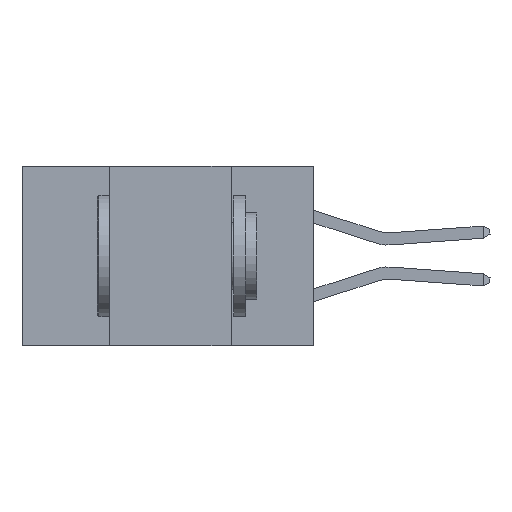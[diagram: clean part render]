
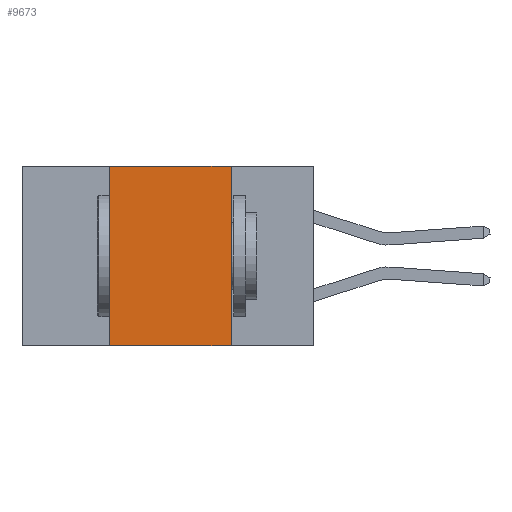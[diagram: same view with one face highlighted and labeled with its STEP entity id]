
A CAD part, left-side view. The second image highlights one B-rep face of the part: STEP entity #9673.
In plain terms, the highlighted planar face has unit normal (-1, 0, 0).
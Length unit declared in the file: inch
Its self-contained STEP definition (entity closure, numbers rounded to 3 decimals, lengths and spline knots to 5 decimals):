
#394 = VERTEX_POINT ( 'NONE', #27516 ) ;
#942 = ORIENTED_EDGE ( 'NONE', *, *, #21760, .F. ) ;
#1142 = DIRECTION ( 'NONE',  ( 1., 0., 0. ) ) ;
#1430 = DIRECTION ( 'NONE',  ( 0., 0., 1. ) ) ;
#1872 = ORIENTED_EDGE ( 'NONE', *, *, #23260, .F. ) ;
#2189 = DIRECTION ( 'NONE',  ( 0., -1., 0. ) ) ;
#4790 = LINE ( 'NONE', #5276, #15573 ) ;
#5215 = EDGE_CURVE ( 'NONE', #14139, #394, #22603, .T. ) ;
#5276 = CARTESIAN_POINT ( 'NONE',  ( 0., 0.6, 0. ) ) ;
#5800 = CARTESIAN_POINT ( 'NONE',  ( 0., 0.42, 0. ) ) ;
#5894 = LINE ( 'NONE', #25523, #15028 ) ;
#6830 = ORIENTED_EDGE ( 'NONE', *, *, #9731, .F. ) ;
#7863 = PLANE ( 'NONE',  #26238 ) ;
#9336 = VERTEX_POINT ( 'NONE', #13077 ) ;
#9538 = VERTEX_POINT ( 'NONE', #9573 ) ;
#9573 = CARTESIAN_POINT ( 'NONE',  ( 0., 0.42, 0. ) ) ;
#9673 = ADVANCED_FACE ( 'NONE', ( #17369 ), #7863, .F. ) ;
#9731 = EDGE_CURVE ( 'NONE', #14139, #9538, #24092, .T. ) ;
#11105 = VECTOR ( 'NONE', #2189, 39.37008 ) ;
#12783 = DIRECTION ( 'NONE',  ( 0., 0., -1. ) ) ;
#13077 = CARTESIAN_POINT ( 'NONE',  ( 0., 0.17, 0. ) ) ;
#14139 = VERTEX_POINT ( 'NONE', #23468 ) ;
#15028 = VECTOR ( 'NONE', #12783, 39.37008 ) ;
#15573 = VECTOR ( 'NONE', #17997, 39.37008 ) ;
#17369 = FACE_OUTER_BOUND ( 'NONE', #21183, .T. ) ;
#17784 = ORIENTED_EDGE ( 'NONE', *, *, #5215, .T. ) ;
#17997 = DIRECTION ( 'NONE',  ( 0., -1., 0. ) ) ;
#21183 = EDGE_LOOP ( 'NONE', ( #942, #1872, #6830, #17784 ) ) ;
#21760 = EDGE_CURVE ( 'NONE', #9336, #394, #5894, .T. ) ;
#22045 = CARTESIAN_POINT ( 'NONE',  ( 0., 0.6, -0.37 ) ) ;
#22603 = LINE ( 'NONE', #22045, #11105 ) ;
#23260 = EDGE_CURVE ( 'NONE', #9538, #9336, #4790, .T. ) ;
#23468 = CARTESIAN_POINT ( 'NONE',  ( 0., 0.42, -0.37 ) ) ;
#24092 = LINE ( 'NONE', #5800, #27512 ) ;
#24863 = DIRECTION ( 'NONE',  ( 0., 0., -1. ) ) ;
#25523 = CARTESIAN_POINT ( 'NONE',  ( 0., 0.17, 0. ) ) ;
#26238 = AXIS2_PLACEMENT_3D ( 'NONE', #27318, #1142, #24863 ) ;
#27318 = CARTESIAN_POINT ( 'NONE',  ( 0., 0.6, 0. ) ) ;
#27512 = VECTOR ( 'NONE', #1430, 39.37008 ) ;
#27516 = CARTESIAN_POINT ( 'NONE',  ( 0., 0.17, -0.37 ) ) ;
